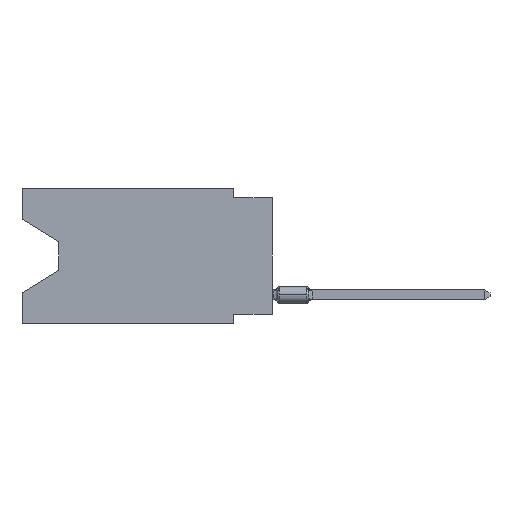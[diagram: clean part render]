
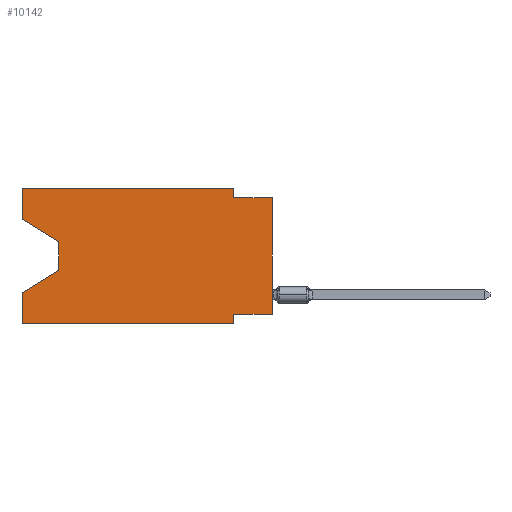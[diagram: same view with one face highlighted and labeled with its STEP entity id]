
A CAD part, left-side view. The second image highlights one B-rep face of the part: STEP entity #10142.
In plain terms, the highlighted planar face has unit normal (-1, 0, 0).
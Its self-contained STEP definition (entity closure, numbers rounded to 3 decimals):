
#362 = VECTOR ( 'NONE', #7808, 1000. ) ;
#504 = LINE ( 'NONE', #7723, #1896 ) ;
#643 = CARTESIAN_POINT ( 'NONE',  ( 0., 16.383, -8.89 ) ) ;
#678 = DIRECTION ( 'NONE',  ( 0., 0., -1. ) ) ;
#812 = VERTEX_POINT ( 'NONE', #5044 ) ;
#1154 = CARTESIAN_POINT ( 'NONE',  ( 0., 16.383, 0. ) ) ;
#1204 = ORIENTED_EDGE ( 'NONE', *, *, #12157, .F. ) ;
#1280 = LINE ( 'NONE', #8518, #6247 ) ;
#1304 = LINE ( 'NONE', #4581, #1349 ) ;
#1349 = VECTOR ( 'NONE', #10858, 1000. ) ;
#1403 = VERTEX_POINT ( 'NONE', #3424 ) ;
#1484 = EDGE_CURVE ( 'NONE', #7388, #11014, #3557, .T. ) ;
#1726 = DIRECTION ( 'NONE',  ( 0., 0., 1. ) ) ;
#1841 = ORIENTED_EDGE ( 'NONE', *, *, #1484, .F. ) ;
#1842 = ORIENTED_EDGE ( 'NONE', *, *, #2076, .T. ) ;
#1896 = VECTOR ( 'NONE', #1726, 1000. ) ;
#2042 = LINE ( 'NONE', #8180, #8286 ) ;
#2076 = EDGE_CURVE ( 'NONE', #4279, #3418, #1280, .T. ) ;
#2087 = DIRECTION ( 'NONE',  ( 0., 1., 0. ) ) ;
#2870 = VERTEX_POINT ( 'NONE', #8663 ) ;
#2922 = ORIENTED_EDGE ( 'NONE', *, *, #8496, .T. ) ;
#3082 = AXIS2_PLACEMENT_3D ( 'NONE', #1154, #8523, #11596 ) ;
#3182 = VERTEX_POINT ( 'NONE', #3968 ) ;
#3250 = ORIENTED_EDGE ( 'NONE', *, *, #13232, .T. ) ;
#3418 = VERTEX_POINT ( 'NONE', #7900 ) ;
#3421 = CARTESIAN_POINT ( 'NONE',  ( 0., 13.97, -3.505 ) ) ;
#3424 = CARTESIAN_POINT ( 'NONE',  ( 0., 16.383, -6.852 ) ) ;
#3500 = VERTEX_POINT ( 'NONE', #13279 ) ;
#3557 = LINE ( 'NONE', #5608, #5626 ) ;
#3695 = ORIENTED_EDGE ( 'NONE', *, *, #6755, .F. ) ;
#3964 = VERTEX_POINT ( 'NONE', #12080 ) ;
#3968 = CARTESIAN_POINT ( 'NONE',  ( 0., 0., -0.635 ) ) ;
#4217 = DIRECTION ( 'NONE',  ( 0., 0., -1. ) ) ;
#4252 = CARTESIAN_POINT ( 'NONE',  ( 0., 16.383, 0. ) ) ;
#4279 = VERTEX_POINT ( 'NONE', #643 ) ;
#4335 = ORIENTED_EDGE ( 'NONE', *, *, #12572, .F. ) ;
#4370 = EDGE_LOOP ( 'NONE', ( #2922, #3250, #13309, #4335, #1842, #9461, #3695, #8381, #8048, #1204, #1841, #5759 ) ) ;
#4424 = FACE_OUTER_BOUND ( 'NONE', #4370, .T. ) ;
#4479 = CARTESIAN_POINT ( 'NONE',  ( 0., 16.383, -2.038 ) ) ;
#4581 = CARTESIAN_POINT ( 'NONE',  ( 0., 16.383, 0. ) ) ;
#4587 = EDGE_CURVE ( 'NONE', #7785, #7388, #1304, .T. ) ;
#4715 = DIRECTION ( 'NONE',  ( 0., 0., -1. ) ) ;
#4755 = CARTESIAN_POINT ( 'NONE',  ( 0., 13.97, -5.385 ) ) ;
#4765 = LINE ( 'NONE', #7025, #7868 ) ;
#5026 = CARTESIAN_POINT ( 'NONE',  ( 0., 0., -8.255 ) ) ;
#5044 = CARTESIAN_POINT ( 'NONE',  ( 0., 13.97, -3.505 ) ) ;
#5067 = DIRECTION ( 'NONE',  ( 0., -0.855, -0.519 ) ) ;
#5232 = EDGE_CURVE ( 'NONE', #7138, #3418, #2042, .T. ) ;
#5608 = CARTESIAN_POINT ( 'NONE',  ( 0., 16.383, 0. ) ) ;
#5626 = VECTOR ( 'NONE', #11070, 1000. ) ;
#5759 = ORIENTED_EDGE ( 'NONE', *, *, #4587, .F. ) ;
#5954 = LINE ( 'NONE', #10116, #11902 ) ;
#6247 = VECTOR ( 'NONE', #11650, 1000. ) ;
#6558 = CARTESIAN_POINT ( 'NONE',  ( 0., 2.54, 0. ) ) ;
#6755 = EDGE_CURVE ( 'NONE', #3964, #7138, #13404, .T. ) ;
#6904 = VECTOR ( 'NONE', #13004, 1000. ) ;
#7018 = EDGE_CURVE ( 'NONE', #2870, #3182, #7885, .T. ) ;
#7025 = CARTESIAN_POINT ( 'NONE',  ( 0., 2.54, 0. ) ) ;
#7132 = CARTESIAN_POINT ( 'NONE',  ( 0., 2.54, -8.255 ) ) ;
#7138 = VERTEX_POINT ( 'NONE', #7132 ) ;
#7388 = VERTEX_POINT ( 'NONE', #4252 ) ;
#7558 = PLANE ( 'NONE',  #3082 ) ;
#7723 = CARTESIAN_POINT ( 'NONE',  ( 0., 0., 0. ) ) ;
#7756 = VECTOR ( 'NONE', #2087, 1000. ) ;
#7785 = VERTEX_POINT ( 'NONE', #4479 ) ;
#7808 = DIRECTION ( 'NONE',  ( 0., -1., 0. ) ) ;
#7831 = EDGE_CURVE ( 'NONE', #3500, #1403, #8984, .T. ) ;
#7868 = VECTOR ( 'NONE', #678, 1000. ) ;
#7885 = LINE ( 'NONE', #8972, #362 ) ;
#7900 = CARTESIAN_POINT ( 'NONE',  ( 0., 2.54, -8.89 ) ) ;
#8048 = ORIENTED_EDGE ( 'NONE', *, *, #7018, .F. ) ;
#8180 = CARTESIAN_POINT ( 'NONE',  ( 0., 2.54, -8.89 ) ) ;
#8286 = VECTOR ( 'NONE', #4217, 1000. ) ;
#8341 = EDGE_CURVE ( 'NONE', #3964, #3182, #504, .T. ) ;
#8381 = ORIENTED_EDGE ( 'NONE', *, *, #8341, .T. ) ;
#8496 = EDGE_CURVE ( 'NONE', #7785, #812, #5954, .T. ) ;
#8518 = CARTESIAN_POINT ( 'NONE',  ( 0., 16.383, -8.89 ) ) ;
#8523 = DIRECTION ( 'NONE',  ( 1., 0., 0. ) ) ;
#8663 = CARTESIAN_POINT ( 'NONE',  ( 0., 2.54, -0.635 ) ) ;
#8972 = CARTESIAN_POINT ( 'NONE',  ( 0., 0., -0.635 ) ) ;
#8984 = LINE ( 'NONE', #4755, #6904 ) ;
#9461 = ORIENTED_EDGE ( 'NONE', *, *, #5232, .F. ) ;
#9932 = DIRECTION ( 'NONE',  ( 0., 0., 1. ) ) ;
#10116 = CARTESIAN_POINT ( 'NONE',  ( 0., 16.383, -2.038 ) ) ;
#10142 = ADVANCED_FACE ( 'NONE', ( #4424 ), #7558, .F. ) ;
#10858 = DIRECTION ( 'NONE',  ( 0., 0., 1. ) ) ;
#10962 = LINE ( 'NONE', #11099, #12852 ) ;
#11014 = VERTEX_POINT ( 'NONE', #6558 ) ;
#11070 = DIRECTION ( 'NONE',  ( 0., -1., 0. ) ) ;
#11099 = CARTESIAN_POINT ( 'NONE',  ( 0., 16.383, 0. ) ) ;
#11596 = DIRECTION ( 'NONE',  ( 0., 0., -1. ) ) ;
#11650 = DIRECTION ( 'NONE',  ( 0., -1., 0. ) ) ;
#11902 = VECTOR ( 'NONE', #5067, 1000. ) ;
#12080 = CARTESIAN_POINT ( 'NONE',  ( 0., 0., -8.255 ) ) ;
#12101 = VECTOR ( 'NONE', #4715, 1000. ) ;
#12157 = EDGE_CURVE ( 'NONE', #11014, #2870, #4765, .T. ) ;
#12572 = EDGE_CURVE ( 'NONE', #4279, #1403, #10962, .T. ) ;
#12762 = LINE ( 'NONE', #3421, #12101 ) ;
#12852 = VECTOR ( 'NONE', #9932, 1000. ) ;
#13004 = DIRECTION ( 'NONE',  ( 0., 0.855, -0.519 ) ) ;
#13232 = EDGE_CURVE ( 'NONE', #812, #3500, #12762, .T. ) ;
#13279 = CARTESIAN_POINT ( 'NONE',  ( 0., 13.97, -5.385 ) ) ;
#13309 = ORIENTED_EDGE ( 'NONE', *, *, #7831, .T. ) ;
#13404 = LINE ( 'NONE', #5026, #7756 ) ;
